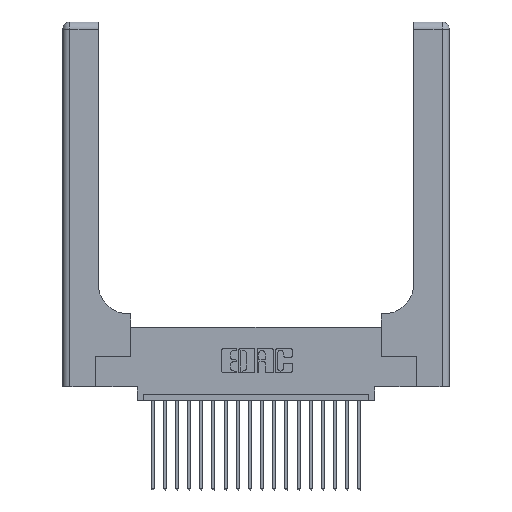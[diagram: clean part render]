
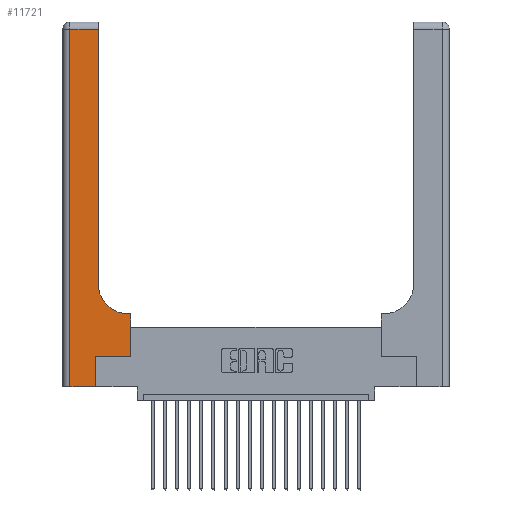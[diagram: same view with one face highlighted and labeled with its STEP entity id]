
A CAD part, top view. The second image highlights one B-rep face of the part: STEP entity #11721.
In plain terms, the highlighted planar face has unit normal (0, 0, 1).
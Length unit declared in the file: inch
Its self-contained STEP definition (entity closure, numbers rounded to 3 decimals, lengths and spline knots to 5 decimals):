
#50 = ORIENTED_EDGE ( 'NONE', *, *, #8706, .T. ) ;
#248 = CARTESIAN_POINT ( 'NONE',  ( 0., 2.94, 0.37 ) ) ;
#612 = DIRECTION ( 'NONE',  ( 0., -1., 0. ) ) ;
#863 = ORIENTED_EDGE ( 'NONE', *, *, #19574, .T. ) ;
#888 = LINE ( 'NONE', #6006, #18489 ) ;
#916 = CARTESIAN_POINT ( 'NONE',  ( 0.5415, 0.6, 0.37 ) ) ;
#1019 = ORIENTED_EDGE ( 'NONE', *, *, #8404, .T. ) ;
#1224 = VECTOR ( 'NONE', #4772, 39.37008 ) ;
#1299 = DIRECTION ( 'NONE',  ( 1., 0., 0. ) ) ;
#2057 = ORIENTED_EDGE ( 'NONE', *, *, #13657, .T. ) ;
#2236 = AXIS2_PLACEMENT_3D ( 'NONE', #9148, #17589, #5519 ) ;
#2444 = VERTEX_POINT ( 'NONE', #3030 ) ;
#2802 = LINE ( 'NONE', #248, #9219 ) ;
#3030 = CARTESIAN_POINT ( 'NONE',  ( 0.2915, 0.85, 0.37 ) ) ;
#3343 = CARTESIAN_POINT ( 'NONE',  ( 0.06, 0., 0.37 ) ) ;
#3581 = AXIS2_PLACEMENT_3D ( 'NONE', #11544, #8108, #1299 ) ;
#3662 = EDGE_CURVE ( 'NONE', #15888, #2444, #14792, .T. ) ;
#3755 = EDGE_CURVE ( 'NONE', #19143, #14166, #888, .T. ) ;
#3870 = CARTESIAN_POINT ( 'NONE',  ( 0.2915, 0.6, 0.37 ) ) ;
#4521 = DIRECTION ( 'NONE',  ( 0., 1., 0. ) ) ;
#4705 = VERTEX_POINT ( 'NONE', #20853 ) ;
#4772 = DIRECTION ( 'NONE',  ( 0., 1., 0. ) ) ;
#4809 = LINE ( 'NONE', #20746, #13508 ) ;
#5299 = ORIENTED_EDGE ( 'NONE', *, *, #3755, .T. ) ;
#5519 = DIRECTION ( 'NONE',  ( -1., 0., 0. ) ) ;
#5576 = VERTEX_POINT ( 'NONE', #3343 ) ;
#5634 = VERTEX_POINT ( 'NONE', #17039 ) ;
#5766 = EDGE_CURVE ( 'NONE', #10438, #5576, #4809, .T. ) ;
#6006 = CARTESIAN_POINT ( 'NONE',  ( 0.5585, 0.25, 0.37 ) ) ;
#6304 = CARTESIAN_POINT ( 'NONE',  ( 0.269, 0., 0.37 ) ) ;
#6736 = LINE ( 'NONE', #3870, #17634 ) ;
#7161 = LINE ( 'NONE', #9185, #10632 ) ;
#8108 = DIRECTION ( 'NONE',  ( 0., 0., -1. ) ) ;
#8383 = CARTESIAN_POINT ( 'NONE',  ( 0.2915, 3., 0.37 ) ) ;
#8404 = EDGE_CURVE ( 'NONE', #2444, #4705, #19365, .T. ) ;
#8706 = EDGE_CURVE ( 'NONE', #14829, #19143, #21476, .T. ) ;
#8932 = ORIENTED_EDGE ( 'NONE', *, *, #15229, .T. ) ;
#9148 = CARTESIAN_POINT ( 'NONE',  ( 0., 3., 0.37 ) ) ;
#9185 = CARTESIAN_POINT ( 'NONE',  ( 0., 0., 0.37 ) ) ;
#9219 = VECTOR ( 'NONE', #15845, 39.37008 ) ;
#9602 = ORIENTED_EDGE ( 'NONE', *, *, #5766, .T. ) ;
#9685 = FACE_OUTER_BOUND ( 'NONE', #18956, .T. ) ;
#10438 = VERTEX_POINT ( 'NONE', #16869 ) ;
#10632 = VECTOR ( 'NONE', #21064, 39.37008 ) ;
#10659 = VECTOR ( 'NONE', #4521, 39.37008 ) ;
#11031 = DIRECTION ( 'NONE',  ( 0., 1., 0. ) ) ;
#11193 = LINE ( 'NONE', #6304, #10659 ) ;
#11544 = CARTESIAN_POINT ( 'NONE',  ( 0.5415, 0.85, 0.37 ) ) ;
#11721 = ADVANCED_FACE ( 'NONE', ( #9685 ), #12408, .F. ) ;
#12385 = CARTESIAN_POINT ( 'NONE',  ( 0.269, 0.25, 0.37 ) ) ;
#12408 = PLANE ( 'NONE',  #2236 ) ;
#13508 = VECTOR ( 'NONE', #612, 39.37008 ) ;
#13643 = DIRECTION ( 'NONE',  ( 1., 0., 0. ) ) ;
#13657 = EDGE_CURVE ( 'NONE', #4705, #10438, #2802, .T. ) ;
#14166 = VERTEX_POINT ( 'NONE', #19026 ) ;
#14434 = CARTESIAN_POINT ( 'NONE',  ( 0.5585, 0.25, 0.37 ) ) ;
#14792 = CIRCLE ( 'NONE', #3581, 0.25 ) ;
#14829 = VERTEX_POINT ( 'NONE', #12385 ) ;
#15108 = VECTOR ( 'NONE', #13643, 39.37008 ) ;
#15229 = EDGE_CURVE ( 'NONE', #14166, #15888, #6736, .T. ) ;
#15845 = DIRECTION ( 'NONE',  ( -1., 0., 0. ) ) ;
#15888 = VERTEX_POINT ( 'NONE', #916 ) ;
#16869 = CARTESIAN_POINT ( 'NONE',  ( 0.06, 2.94, 0.37 ) ) ;
#17003 = CARTESIAN_POINT ( 'NONE',  ( 0.269, 0.25, 0.37 ) ) ;
#17039 = CARTESIAN_POINT ( 'NONE',  ( 0.269, 0., 0.37 ) ) ;
#17589 = DIRECTION ( 'NONE',  ( 0., 0., -1. ) ) ;
#17634 = VECTOR ( 'NONE', #18919, 39.37008 ) ;
#18489 = VECTOR ( 'NONE', #11031, 39.37008 ) ;
#18919 = DIRECTION ( 'NONE',  ( -1., 0., 0. ) ) ;
#18956 = EDGE_LOOP ( 'NONE', ( #1019, #2057, #9602, #863, #19000, #50, #5299, #8932, #21397 ) ) ;
#19000 = ORIENTED_EDGE ( 'NONE', *, *, #19774, .T. ) ;
#19026 = CARTESIAN_POINT ( 'NONE',  ( 0.5585, 0.6, 0.37 ) ) ;
#19143 = VERTEX_POINT ( 'NONE', #14434 ) ;
#19365 = LINE ( 'NONE', #8383, #1224 ) ;
#19574 = EDGE_CURVE ( 'NONE', #5576, #5634, #7161, .T. ) ;
#19774 = EDGE_CURVE ( 'NONE', #5634, #14829, #11193, .T. ) ;
#20746 = CARTESIAN_POINT ( 'NONE',  ( 0.06, 3., 0.37 ) ) ;
#20853 = CARTESIAN_POINT ( 'NONE',  ( 0.2915, 2.94, 0.37 ) ) ;
#21064 = DIRECTION ( 'NONE',  ( 1., 0., 0. ) ) ;
#21397 = ORIENTED_EDGE ( 'NONE', *, *, #3662, .T. ) ;
#21476 = LINE ( 'NONE', #17003, #15108 ) ;
